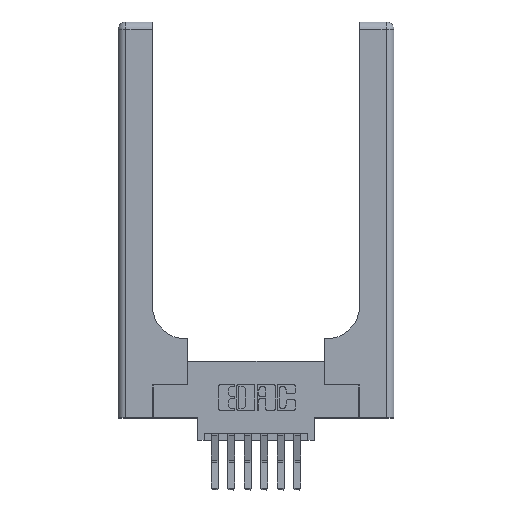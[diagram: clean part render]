
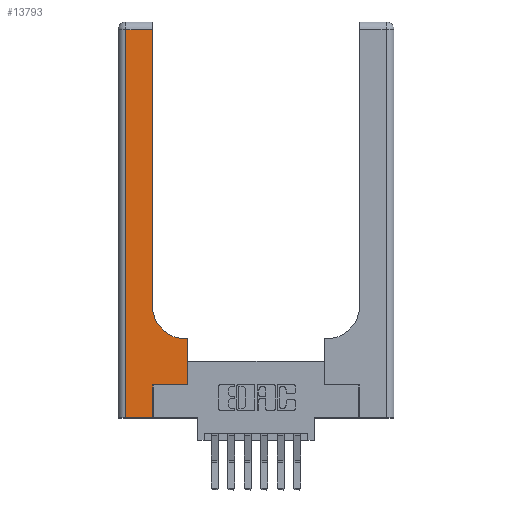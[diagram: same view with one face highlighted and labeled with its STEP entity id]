
A CAD part, top view. The second image highlights one B-rep face of the part: STEP entity #13793.
In plain terms, the highlighted planar face has unit normal (0, 0, 1).
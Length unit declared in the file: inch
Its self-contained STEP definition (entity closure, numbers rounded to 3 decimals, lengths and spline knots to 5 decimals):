
#179 = EDGE_CURVE ( 'NONE', #12869, #12278, #10287, .T. ) ;
#247 = CARTESIAN_POINT ( 'NONE',  ( 0.265, 0.25, 0.37 ) ) ;
#468 = LINE ( 'NONE', #247, #2403 ) ;
#588 = ORIENTED_EDGE ( 'NONE', *, *, #14556, .T. ) ;
#668 = CARTESIAN_POINT ( 'NONE',  ( 0.26, 2.94, 0.37 ) ) ;
#1034 = CARTESIAN_POINT ( 'NONE',  ( 0., 3., 0.37 ) ) ;
#1202 = DIRECTION ( 'NONE',  ( 1., 0., 0. ) ) ;
#1229 = CIRCLE ( 'NONE', #1468, 0.25 ) ;
#1270 = CARTESIAN_POINT ( 'NONE',  ( 0.528, 0.25, 0.37 ) ) ;
#1310 = CARTESIAN_POINT ( 'NONE',  ( 0.528, 0.25, 0.37 ) ) ;
#1452 = VERTEX_POINT ( 'NONE', #12829 ) ;
#1468 = AXIS2_PLACEMENT_3D ( 'NONE', #10717, #12941, #8492 ) ;
#1534 = DIRECTION ( 'NONE',  ( 0., 1., 0. ) ) ;
#1732 = ORIENTED_EDGE ( 'NONE', *, *, #11042, .T. ) ;
#1817 = CARTESIAN_POINT ( 'NONE',  ( 0.265, 0., 0.37 ) ) ;
#1895 = VECTOR ( 'NONE', #7718, 39.37008 ) ;
#2403 = VECTOR ( 'NONE', #9266, 39.37008 ) ;
#2417 = CARTESIAN_POINT ( 'NONE',  ( 0.265, 0., 0.37 ) ) ;
#2902 = VECTOR ( 'NONE', #11597, 39.37008 ) ;
#2987 = CARTESIAN_POINT ( 'NONE',  ( 0.51, 0.6, 0.37 ) ) ;
#3022 = VERTEX_POINT ( 'NONE', #12620 ) ;
#3186 = EDGE_CURVE ( 'NONE', #12278, #3022, #13336, .T. ) ;
#3218 = CARTESIAN_POINT ( 'NONE',  ( 0., 2.94, 0.37 ) ) ;
#3349 = CARTESIAN_POINT ( 'NONE',  ( 0.26, 3., 0.37 ) ) ;
#3833 = VECTOR ( 'NONE', #1202, 39.37008 ) ;
#4410 = CARTESIAN_POINT ( 'NONE',  ( 0.26, 0.85, 0.37 ) ) ;
#4422 = DIRECTION ( 'NONE',  ( -1., 0., 0. ) ) ;
#4432 = ORIENTED_EDGE ( 'NONE', *, *, #10405, .T. ) ;
#4453 = LINE ( 'NONE', #7994, #3833 ) ;
#4695 = EDGE_CURVE ( 'NONE', #1452, #14314, #468, .T. ) ;
#5010 = VECTOR ( 'NONE', #1534, 39.37008 ) ;
#5046 = VECTOR ( 'NONE', #11304, 39.37008 ) ;
#5130 = EDGE_CURVE ( 'NONE', #5608, #12869, #1229, .T. ) ;
#5252 = LINE ( 'NONE', #6133, #8782 ) ;
#5608 = VERTEX_POINT ( 'NONE', #2987 ) ;
#6133 = CARTESIAN_POINT ( 'NONE',  ( 0.06, 3., 0.37 ) ) ;
#6796 = DIRECTION ( 'NONE',  ( 0., -1., 0. ) ) ;
#7026 = LINE ( 'NONE', #1270, #5046 ) ;
#7088 = CARTESIAN_POINT ( 'NONE',  ( 0.26, 0.6, 0.37 ) ) ;
#7103 = ORIENTED_EDGE ( 'NONE', *, *, #4695, .T. ) ;
#7549 = ORIENTED_EDGE ( 'NONE', *, *, #13015, .T. ) ;
#7718 = DIRECTION ( 'NONE',  ( -1., 0., 0. ) ) ;
#7994 = CARTESIAN_POINT ( 'NONE',  ( 0., 0., 0.37 ) ) ;
#8018 = ORIENTED_EDGE ( 'NONE', *, *, #179, .T. ) ;
#8028 = PLANE ( 'NONE',  #14231 ) ;
#8194 = LINE ( 'NONE', #7088, #2902 ) ;
#8492 = DIRECTION ( 'NONE',  ( 1., 0., 0. ) ) ;
#8782 = VECTOR ( 'NONE', #6796, 39.37008 ) ;
#8996 = FACE_OUTER_BOUND ( 'NONE', #13598, .T. ) ;
#9150 = DIRECTION ( 'NONE',  ( 0., 0., -1. ) ) ;
#9266 = DIRECTION ( 'NONE',  ( 1., 0., 0. ) ) ;
#10061 = CARTESIAN_POINT ( 'NONE',  ( 0.528, 0.6, 0.37 ) ) ;
#10071 = DIRECTION ( 'NONE',  ( 0., 1., 0. ) ) ;
#10091 = CARTESIAN_POINT ( 'NONE',  ( 0.06, 0., 0.37 ) ) ;
#10287 = LINE ( 'NONE', #3349, #11485 ) ;
#10405 = EDGE_CURVE ( 'NONE', #12766, #12956, #4453, .T. ) ;
#10717 = CARTESIAN_POINT ( 'NONE',  ( 0.51, 0.85, 0.37 ) ) ;
#10829 = EDGE_CURVE ( 'NONE', #3022, #12766, #5252, .T. ) ;
#11030 = ORIENTED_EDGE ( 'NONE', *, *, #3186, .T. ) ;
#11042 = EDGE_CURVE ( 'NONE', #14445, #5608, #8194, .T. ) ;
#11304 = DIRECTION ( 'NONE',  ( 0., 1., 0. ) ) ;
#11485 = VECTOR ( 'NONE', #10071, 39.37008 ) ;
#11597 = DIRECTION ( 'NONE',  ( -1., 0., 0. ) ) ;
#12278 = VERTEX_POINT ( 'NONE', #668 ) ;
#12620 = CARTESIAN_POINT ( 'NONE',  ( 0.06, 2.94, 0.37 ) ) ;
#12766 = VERTEX_POINT ( 'NONE', #10091 ) ;
#12829 = CARTESIAN_POINT ( 'NONE',  ( 0.265, 0.25, 0.37 ) ) ;
#12869 = VERTEX_POINT ( 'NONE', #4410 ) ;
#12941 = DIRECTION ( 'NONE',  ( 0., 0., -1. ) ) ;
#12956 = VERTEX_POINT ( 'NONE', #2417 ) ;
#13015 = EDGE_CURVE ( 'NONE', #12956, #1452, #13924, .T. ) ;
#13336 = LINE ( 'NONE', #3218, #1895 ) ;
#13398 = ORIENTED_EDGE ( 'NONE', *, *, #5130, .T. ) ;
#13598 = EDGE_LOOP ( 'NONE', ( #8018, #11030, #14436, #4432, #7549, #7103, #588, #1732, #13398 ) ) ;
#13793 = ADVANCED_FACE ( 'NONE', ( #8996 ), #8028, .F. ) ;
#13924 = LINE ( 'NONE', #1817, #5010 ) ;
#14231 = AXIS2_PLACEMENT_3D ( 'NONE', #1034, #9150, #4422 ) ;
#14314 = VERTEX_POINT ( 'NONE', #1310 ) ;
#14436 = ORIENTED_EDGE ( 'NONE', *, *, #10829, .T. ) ;
#14445 = VERTEX_POINT ( 'NONE', #10061 ) ;
#14556 = EDGE_CURVE ( 'NONE', #14314, #14445, #7026, .T. ) ;
